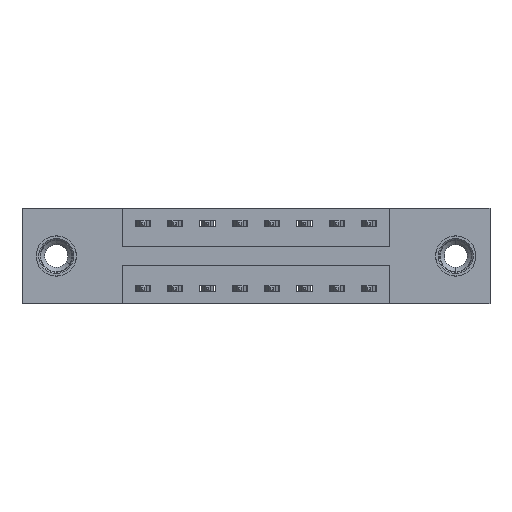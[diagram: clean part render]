
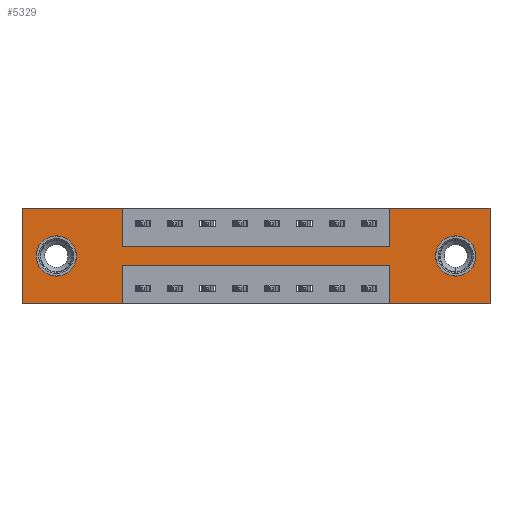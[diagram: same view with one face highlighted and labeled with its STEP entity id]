
A CAD part, front view. The second image highlights one B-rep face of the part: STEP entity #5329.
In plain terms, the highlighted planar face has unit normal (0, -1, 0).
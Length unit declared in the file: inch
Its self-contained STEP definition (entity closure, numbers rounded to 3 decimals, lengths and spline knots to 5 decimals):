
#95 = CARTESIAN_POINT ( 'NONE',  ( 0., 0., 0. ) ) ;
#98 = CARTESIAN_POINT ( 'NONE',  ( 1.81, 0., -0.37 ) ) ;
#112 = ORIENTED_EDGE ( 'NONE', *, *, #10953, .F. ) ;
#308 = CARTESIAN_POINT ( 'NONE',  ( 0.3875, 0., 0. ) ) ;
#403 = VERTEX_POINT ( 'NONE', #8603 ) ;
#411 = EDGE_CURVE ( 'NONE', #2118, #4406, #4440, .T. ) ;
#470 = AXIS2_PLACEMENT_3D ( 'NONE', #1350, #10816, #635 ) ;
#492 = CARTESIAN_POINT ( 'NONE',  ( 0.1325, 0., -0.185 ) ) ;
#507 = CARTESIAN_POINT ( 'NONE',  ( 0., 0., -0.37 ) ) ;
#515 = VERTEX_POINT ( 'NONE', #10475 ) ;
#565 = VECTOR ( 'NONE', #2001, 39.37008 ) ;
#635 = DIRECTION ( 'NONE',  ( 0., 0., -1. ) ) ;
#681 = VECTOR ( 'NONE', #10508, 39.37008 ) ;
#778 = EDGE_CURVE ( 'NONE', #9945, #7675, #6702, .T. ) ;
#917 = EDGE_LOOP ( 'NONE', ( #4450, #2822 ) ) ;
#971 = DIRECTION ( 'NONE',  ( 0., 1., 0. ) ) ;
#1205 = FACE_BOUND ( 'NONE', #2355, .T. ) ;
#1237 = EDGE_CURVE ( 'NONE', #6425, #7520, #9668, .T. ) ;
#1293 = DIRECTION ( 'NONE',  ( 0., 1., 0. ) ) ;
#1344 = EDGE_CURVE ( 'NONE', #2442, #9162, #7946, .T. ) ;
#1350 = CARTESIAN_POINT ( 'NONE',  ( 0., 0., -0.37 ) ) ;
#1470 = CARTESIAN_POINT ( 'NONE',  ( 1.4225, 0., -0.15 ) ) ;
#1500 = VERTEX_POINT ( 'NONE', #10127 ) ;
#1536 = AXIS2_PLACEMENT_3D ( 'NONE', #6108, #971, #4268 ) ;
#1619 = DIRECTION ( 'NONE',  ( 0., 0., 1. ) ) ;
#1936 = CARTESIAN_POINT ( 'NONE',  ( 0., 0., -0.37 ) ) ;
#2001 = DIRECTION ( 'NONE',  ( 0., 0., 1. ) ) ;
#2107 = CIRCLE ( 'NONE', #5983, 0.078 ) ;
#2118 = VERTEX_POINT ( 'NONE', #308 ) ;
#2122 = DIRECTION ( 'NONE',  ( 1., 0., 0. ) ) ;
#2177 = PLANE ( 'NONE',  #470 ) ;
#2345 = ORIENTED_EDGE ( 'NONE', *, *, #2959, .F. ) ;
#2355 = EDGE_LOOP ( 'NONE', ( #11005, #6950 ) ) ;
#2442 = VERTEX_POINT ( 'NONE', #10390 ) ;
#2596 = EDGE_CURVE ( 'NONE', #7675, #9945, #10030, .T. ) ;
#2721 = ORIENTED_EDGE ( 'NONE', *, *, #5926, .F. ) ;
#2822 = ORIENTED_EDGE ( 'NONE', *, *, #2596, .T. ) ;
#2832 = VERTEX_POINT ( 'NONE', #9302 ) ;
#2959 = EDGE_CURVE ( 'NONE', #10226, #1500, #9519, .T. ) ;
#3101 = CARTESIAN_POINT ( 'NONE',  ( 1.4225, 0., 0. ) ) ;
#3247 = EDGE_CURVE ( 'NONE', #1500, #2442, #3433, .T. ) ;
#3266 = ORIENTED_EDGE ( 'NONE', *, *, #7591, .F. ) ;
#3344 = DIRECTION ( 'NONE',  ( 0., 0., -1. ) ) ;
#3433 = LINE ( 'NONE', #3736, #565 ) ;
#3522 = EDGE_CURVE ( 'NONE', #3800, #5333, #7649, .T. ) ;
#3531 = CARTESIAN_POINT ( 'NONE',  ( 1.81, 0., 0. ) ) ;
#3735 = LINE ( 'NONE', #1936, #5602 ) ;
#3736 = CARTESIAN_POINT ( 'NONE',  ( 1.4225, 0., -0.37 ) ) ;
#3800 = VERTEX_POINT ( 'NONE', #1470 ) ;
#3864 = LINE ( 'NONE', #5727, #8330 ) ;
#3955 = DIRECTION ( 'NONE',  ( 0., 0., -1. ) ) ;
#3967 = CARTESIAN_POINT ( 'NONE',  ( 0., 0., 0. ) ) ;
#4072 = ORIENTED_EDGE ( 'NONE', *, *, #3522, .F. ) ;
#4107 = DIRECTION ( 'NONE',  ( 0., 1., 0. ) ) ;
#4226 = CARTESIAN_POINT ( 'NONE',  ( 0.1325, 0., -0.263 ) ) ;
#4268 = DIRECTION ( 'NONE',  ( 0., 0., 1. ) ) ;
#4292 = LINE ( 'NONE', #7259, #4829 ) ;
#4406 = VERTEX_POINT ( 'NONE', #8534 ) ;
#4440 = LINE ( 'NONE', #7824, #681 ) ;
#4450 = ORIENTED_EDGE ( 'NONE', *, *, #778, .T. ) ;
#4558 = CARTESIAN_POINT ( 'NONE',  ( 1.4225, 0., 0. ) ) ;
#4714 = AXIS2_PLACEMENT_3D ( 'NONE', #492, #9077, #5691 ) ;
#4728 = ORIENTED_EDGE ( 'NONE', *, *, #1237, .F. ) ;
#4829 = VECTOR ( 'NONE', #2122, 39.37008 ) ;
#4869 = VECTOR ( 'NONE', #9914, 39.37008 ) ;
#4927 = ORIENTED_EDGE ( 'NONE', *, *, #8342, .F. ) ;
#4974 = ORIENTED_EDGE ( 'NONE', *, *, #8892, .F. ) ;
#5073 = LINE ( 'NONE', #8930, #9438 ) ;
#5138 = DIRECTION ( 'NONE',  ( 1., 0., 0. ) ) ;
#5329 = ADVANCED_FACE ( 'NONE', ( #1205, #7621, #5379 ), #2177, .T. ) ;
#5333 = VERTEX_POINT ( 'NONE', #3101 ) ;
#5337 = AXIS2_PLACEMENT_3D ( 'NONE', #5593, #1293, #10066 ) ;
#5367 = ORIENTED_EDGE ( 'NONE', *, *, #7423, .F. ) ;
#5379 = FACE_OUTER_BOUND ( 'NONE', #9280, .T. ) ;
#5593 = CARTESIAN_POINT ( 'NONE',  ( 1.6775, 0., -0.185 ) ) ;
#5602 = VECTOR ( 'NONE', #7956, 39.37008 ) ;
#5691 = DIRECTION ( 'NONE',  ( 0., 0., 1. ) ) ;
#5727 = CARTESIAN_POINT ( 'NONE',  ( 1.81, 0., 0. ) ) ;
#5926 = EDGE_CURVE ( 'NONE', #4406, #3800, #4292, .T. ) ;
#5983 = AXIS2_PLACEMENT_3D ( 'NONE', #8231, #4107, #8335 ) ;
#6108 = CARTESIAN_POINT ( 'NONE',  ( 0.1325, 0., -0.185 ) ) ;
#6363 = ORIENTED_EDGE ( 'NONE', *, *, #3247, .F. ) ;
#6425 = VERTEX_POINT ( 'NONE', #10542 ) ;
#6480 = DIRECTION ( 'NONE',  ( -1., 0., 0. ) ) ;
#6630 = CIRCLE ( 'NONE', #5337, 0.078 ) ;
#6672 = EDGE_CURVE ( 'NONE', #515, #403, #2107, .T. ) ;
#6702 = CIRCLE ( 'NONE', #1536, 0.078 ) ;
#6731 = LINE ( 'NONE', #3967, #4869 ) ;
#6795 = VECTOR ( 'NONE', #1619, 39.37008 ) ;
#6950 = ORIENTED_EDGE ( 'NONE', *, *, #6672, .T. ) ;
#7054 = VECTOR ( 'NONE', #6480, 39.37008 ) ;
#7259 = CARTESIAN_POINT ( 'NONE',  ( 0.3875, 0., -0.15 ) ) ;
#7423 = EDGE_CURVE ( 'NONE', #7520, #2118, #10859, .T. ) ;
#7429 = CARTESIAN_POINT ( 'NONE',  ( 0., 0., 0. ) ) ;
#7520 = VERTEX_POINT ( 'NONE', #95 ) ;
#7591 = EDGE_CURVE ( 'NONE', #9162, #2832, #5073, .T. ) ;
#7593 = CARTESIAN_POINT ( 'NONE',  ( 0.1325, 0., -0.107 ) ) ;
#7621 = FACE_BOUND ( 'NONE', #917, .T. ) ;
#7649 = LINE ( 'NONE', #4558, #10282 ) ;
#7661 = VECTOR ( 'NONE', #9886, 39.37008 ) ;
#7675 = VERTEX_POINT ( 'NONE', #4226 ) ;
#7691 = CARTESIAN_POINT ( 'NONE',  ( 0.3875, 0., -0.22 ) ) ;
#7824 = CARTESIAN_POINT ( 'NONE',  ( 0.3875, 0., 0. ) ) ;
#7946 = LINE ( 'NONE', #7691, #7054 ) ;
#7956 = DIRECTION ( 'NONE',  ( -1., 0., 0. ) ) ;
#8231 = CARTESIAN_POINT ( 'NONE',  ( 1.6775, 0., -0.185 ) ) ;
#8330 = VECTOR ( 'NONE', #3955, 39.37008 ) ;
#8335 = DIRECTION ( 'NONE',  ( 0., 0., -1. ) ) ;
#8342 = EDGE_CURVE ( 'NONE', #10585, #10226, #3864, .T. ) ;
#8389 = ORIENTED_EDGE ( 'NONE', *, *, #1344, .F. ) ;
#8534 = CARTESIAN_POINT ( 'NONE',  ( 0.3875, 0., -0.15 ) ) ;
#8590 = VECTOR ( 'NONE', #5138, 39.37008 ) ;
#8603 = CARTESIAN_POINT ( 'NONE',  ( 1.6775, 0., -0.107 ) ) ;
#8892 = EDGE_CURVE ( 'NONE', #2832, #6425, #3735, .T. ) ;
#8930 = CARTESIAN_POINT ( 'NONE',  ( 0.3875, 0., -0.37 ) ) ;
#9077 = DIRECTION ( 'NONE',  ( 0., 1., 0. ) ) ;
#9162 = VERTEX_POINT ( 'NONE', #9375 ) ;
#9280 = EDGE_LOOP ( 'NONE', ( #3266, #8389, #6363, #2345, #4927, #112, #4072, #2721, #10722, #5367, #4728, #4974 ) ) ;
#9302 = CARTESIAN_POINT ( 'NONE',  ( 0.3875, 0., -0.37 ) ) ;
#9375 = CARTESIAN_POINT ( 'NONE',  ( 0.3875, 0., -0.22 ) ) ;
#9438 = VECTOR ( 'NONE', #3344, 39.37008 ) ;
#9519 = LINE ( 'NONE', #507, #7661 ) ;
#9668 = LINE ( 'NONE', #9826, #6795 ) ;
#9826 = CARTESIAN_POINT ( 'NONE',  ( 0., 0., 0. ) ) ;
#9886 = DIRECTION ( 'NONE',  ( -1., 0., 0. ) ) ;
#9914 = DIRECTION ( 'NONE',  ( 1., 0., 0. ) ) ;
#9945 = VERTEX_POINT ( 'NONE', #7593 ) ;
#10030 = CIRCLE ( 'NONE', #4714, 0.078 ) ;
#10052 = EDGE_CURVE ( 'NONE', #403, #515, #6630, .T. ) ;
#10066 = DIRECTION ( 'NONE',  ( 0., 0., -1. ) ) ;
#10127 = CARTESIAN_POINT ( 'NONE',  ( 1.4225, 0., -0.37 ) ) ;
#10226 = VERTEX_POINT ( 'NONE', #98 ) ;
#10282 = VECTOR ( 'NONE', #10600, 39.37008 ) ;
#10390 = CARTESIAN_POINT ( 'NONE',  ( 1.4225, 0., -0.22 ) ) ;
#10475 = CARTESIAN_POINT ( 'NONE',  ( 1.6775, 0., -0.263 ) ) ;
#10508 = DIRECTION ( 'NONE',  ( 0., 0., -1. ) ) ;
#10542 = CARTESIAN_POINT ( 'NONE',  ( 0., 0., -0.37 ) ) ;
#10585 = VERTEX_POINT ( 'NONE', #3531 ) ;
#10600 = DIRECTION ( 'NONE',  ( 0., 0., 1. ) ) ;
#10722 = ORIENTED_EDGE ( 'NONE', *, *, #411, .F. ) ;
#10816 = DIRECTION ( 'NONE',  ( 0., -1., 0. ) ) ;
#10859 = LINE ( 'NONE', #7429, #8590 ) ;
#10953 = EDGE_CURVE ( 'NONE', #5333, #10585, #6731, .T. ) ;
#11005 = ORIENTED_EDGE ( 'NONE', *, *, #10052, .T. ) ;
